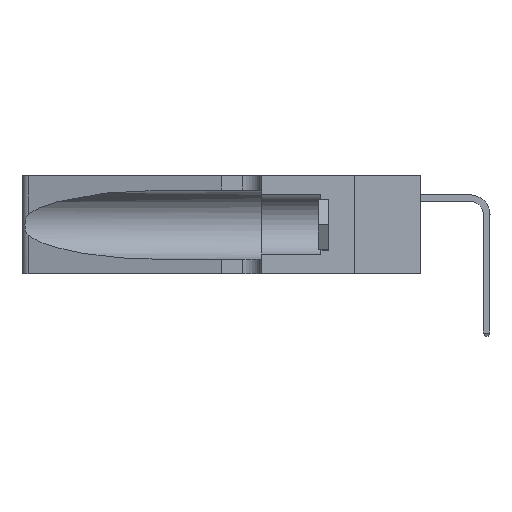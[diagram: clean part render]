
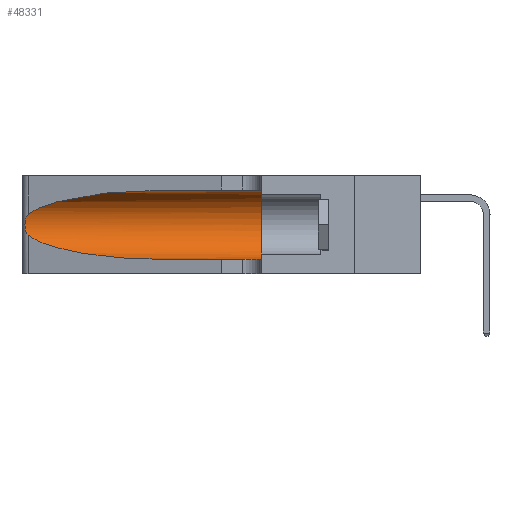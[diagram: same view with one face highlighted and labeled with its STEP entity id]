
A CAD part, left-side view. The second image highlights one B-rep face of the part: STEP entity #48331.
In plain terms, the highlighted cylindrical face has radius 3.308 mm (diameter 6.617 mm), a partial arc.
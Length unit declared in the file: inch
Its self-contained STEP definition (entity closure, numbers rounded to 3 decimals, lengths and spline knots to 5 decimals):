
#387 = CARTESIAN_POINT ( 'NONE',  ( 0.18966, 0.96281, 0.31525 ) ) ;
#763 = ORIENTED_EDGE ( 'NONE', *, *, #46817, .F. ) ;
#946 = CARTESIAN_POINT ( 'NONE',  ( 0.1305, 1.61858, 0.31525 ) ) ;
#2245 = LINE ( 'NONE', #13937, #11605 ) ;
#2256 = CARTESIAN_POINT ( 'NONE',  ( 0.1305, 0.72297, 0.05475 ) ) ;
#2976 =( BOUNDED_CURVE ( )  B_SPLINE_CURVE ( 3, ( #18150, #22179, #26205, #2256 ),
 .UNSPECIFIED., .F., .F. ) 
 B_SPLINE_CURVE_WITH_KNOTS ( ( 4, 4 ),
 ( 3.44316, 4.71239 ),
 .UNSPECIFIED. ) 
 CURVE ( )  GEOMETRIC_REPRESENTATION_ITEM ( )  RATIONAL_B_SPLINE_CURVE ( ( 1., 0.87, 0.87, 1. ) ) 
 REPRESENTATION_ITEM ( '' )  );
#3508 = CARTESIAN_POINT ( 'NONE',  ( 0.26017, 1.23833, 0.17102 ) ) ;
#4798 = VERTEX_POINT ( 'NONE', #8925 ) ;
#5767 = VECTOR ( 'NONE', #40823, 39.37008 ) ;
#7537 = CARTESIAN_POINT ( 'NONE',  ( 0.25789, 1.23486, 0.15765 ) ) ;
#8399 = CARTESIAN_POINT ( 'NONE',  ( 0.1305, 0.35, 0.31525 ) ) ;
#8925 = CARTESIAN_POINT ( 'NONE',  ( 0.25487, 1.22718, 0.22369 ) ) ;
#11538 = CARTESIAN_POINT ( 'NONE',  ( 0.25555, 1.22993, 0.14849 ) ) ;
#11556 = ORIENTED_EDGE ( 'NONE', *, *, #31019, .F. ) ;
#11605 = VECTOR ( 'NONE', #18130, 39.37008 ) ;
#11637 = VERTEX_POINT ( 'NONE', #12142 ) ;
#12142 = CARTESIAN_POINT ( 'NONE',  ( 0.25487, 1.22718, 0.14631 ) ) ;
#12671 = VERTEX_POINT ( 'NONE', #25420 ) ;
#13937 = CARTESIAN_POINT ( 'NONE',  ( 0.1305, 1.61858, 0.05475 ) ) ;
#16449 = CARTESIAN_POINT ( 'NONE',  ( 0.2373, 1.15595, 0.28018 ) ) ;
#17163 = AXIS2_PLACEMENT_3D ( 'NONE', #42837, #34863, #26739 ) ;
#17323 = EDGE_CURVE ( 'NONE', #4798, #11637, #34793, .T. ) ;
#18130 = DIRECTION ( 'NONE',  ( 0., -1., 0. ) ) ;
#18150 = CARTESIAN_POINT ( 'NONE',  ( 0.25487, 1.22718, 0.14631 ) ) ;
#19412 = CARTESIAN_POINT ( 'NONE',  ( 0.25787, 1.23484, 0.2124 ) ) ;
#20995 = DIRECTION ( 'NONE',  ( 0., 1., 0. ) ) ;
#21200 = CIRCLE ( 'NONE', #27530, 0.13025 ) ;
#21467 = EDGE_CURVE ( 'NONE', #12671, #37685, #2245, .T. ) ;
#21569 =( BOUNDED_CURVE ( )  B_SPLINE_CURVE ( 3, ( #28345, #387, #16449, #44413 ),
 .UNSPECIFIED., .F., .F. ) 
 B_SPLINE_CURVE_WITH_KNOTS ( ( 4, 4 ),
 ( 1.5708, 2.84003 ),
 .UNSPECIFIED. ) 
 CURVE ( )  GEOMETRIC_REPRESENTATION_ITEM ( )  RATIONAL_B_SPLINE_CURVE ( ( 1., 0.87, 0.87, 1. ) ) 
 REPRESENTATION_ITEM ( '' )  );
#21998 = CARTESIAN_POINT ( 'NONE',  ( 0.1305, 0.72297, 0.31525 ) ) ;
#22179 = CARTESIAN_POINT ( 'NONE',  ( 0.2373, 1.15595, 0.08982 ) ) ;
#22221 = ORIENTED_EDGE ( 'NONE', *, *, #51298, .T. ) ;
#22732 = EDGE_LOOP ( 'NONE', ( #42030, #27302, #22221, #28213, #763, #11556 ) ) ;
#23454 = CARTESIAN_POINT ( 'NONE',  ( 0.26018, 1.23835, 0.19895 ) ) ;
#25420 = CARTESIAN_POINT ( 'NONE',  ( 0.1305, 0.72297, 0.05475 ) ) ;
#26205 = CARTESIAN_POINT ( 'NONE',  ( 0.18966, 0.96281, 0.05475 ) ) ;
#26739 = DIRECTION ( 'NONE',  ( 0., 0., -1. ) ) ;
#27302 = ORIENTED_EDGE ( 'NONE', *, *, #17323, .T. ) ;
#27472 = CARTESIAN_POINT ( 'NONE',  ( 0.26075, 1.23896, 0.178 ) ) ;
#27530 = AXIS2_PLACEMENT_3D ( 'NONE', #44936, #20995, #48953 ) ;
#28213 = ORIENTED_EDGE ( 'NONE', *, *, #21467, .T. ) ;
#28345 = CARTESIAN_POINT ( 'NONE',  ( 0.1305, 0.72297, 0.31525 ) ) ;
#31019 = EDGE_CURVE ( 'NONE', #33410, #35013, #48285, .T. ) ;
#31547 = CARTESIAN_POINT ( 'NONE',  ( 0.25856, 1.23593, 0.16098 ) ) ;
#33410 = VERTEX_POINT ( 'NONE', #21998 ) ;
#34793 = B_SPLINE_CURVE_WITH_KNOTS ( 'NONE', 3,
 ( #51214, #39206, #43373, #19412, #47371, #23454, #51389, #27472, #3508, #31547, #7537, #35593, #11538, #39544 ),
 .UNSPECIFIED., .F., .F.,
 ( 4, 2, 2, 2, 2, 2, 4 ),
 ( 0., 0.00027, 0.00053, 0.00107, 0.0016, 0.00187, 0.00214 ),
 .UNSPECIFIED. ) ;
#34863 = DIRECTION ( 'NONE',  ( 0., -1., 0. ) ) ;
#35013 = VERTEX_POINT ( 'NONE', #8399 ) ;
#35398 = CARTESIAN_POINT ( 'NONE',  ( 0.1305, 0.35, 0.05475 ) ) ;
#35593 = CARTESIAN_POINT ( 'NONE',  ( 0.25639, 1.23186, 0.15144 ) ) ;
#37685 = VERTEX_POINT ( 'NONE', #35398 ) ;
#39206 = CARTESIAN_POINT ( 'NONE',  ( 0.25555, 1.22994, 0.2215 ) ) ;
#39544 = CARTESIAN_POINT ( 'NONE',  ( 0.25487, 1.22718, 0.14631 ) ) ;
#40449 = CYLINDRICAL_SURFACE ( 'NONE', #17163, 0.13025 ) ;
#40823 = DIRECTION ( 'NONE',  ( 0., -1., 0. ) ) ;
#41696 = FACE_OUTER_BOUND ( 'NONE', #22732, .T. ) ;
#42030 = ORIENTED_EDGE ( 'NONE', *, *, #44454, .T. ) ;
#42837 = CARTESIAN_POINT ( 'NONE',  ( 0.1305, 1.61858, 0.185 ) ) ;
#43373 = CARTESIAN_POINT ( 'NONE',  ( 0.25639, 1.23184, 0.21858 ) ) ;
#44413 = CARTESIAN_POINT ( 'NONE',  ( 0.25487, 1.22718, 0.22369 ) ) ;
#44454 = EDGE_CURVE ( 'NONE', #33410, #4798, #21569, .T. ) ;
#44936 = CARTESIAN_POINT ( 'NONE',  ( 0.1305, 0.35, 0.185 ) ) ;
#46817 = EDGE_CURVE ( 'NONE', #35013, #37685, #21200, .T. ) ;
#47371 = CARTESIAN_POINT ( 'NONE',  ( 0.25854, 1.2359, 0.20912 ) ) ;
#48285 = LINE ( 'NONE', #946, #5767 ) ;
#48331 = ADVANCED_FACE ( 'NONE', ( #41696 ), #40449, .F. ) ;
#48953 = DIRECTION ( 'NONE',  ( 0., 0., 1. ) ) ;
#51214 = CARTESIAN_POINT ( 'NONE',  ( 0.25487, 1.22718, 0.22369 ) ) ;
#51298 = EDGE_CURVE ( 'NONE', #11637, #12671, #2976, .T. ) ;
#51389 = CARTESIAN_POINT ( 'NONE',  ( 0.26075, 1.23896, 0.19203 ) ) ;
